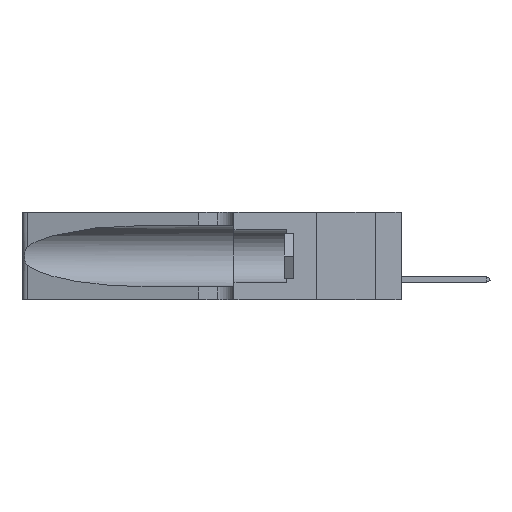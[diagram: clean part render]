
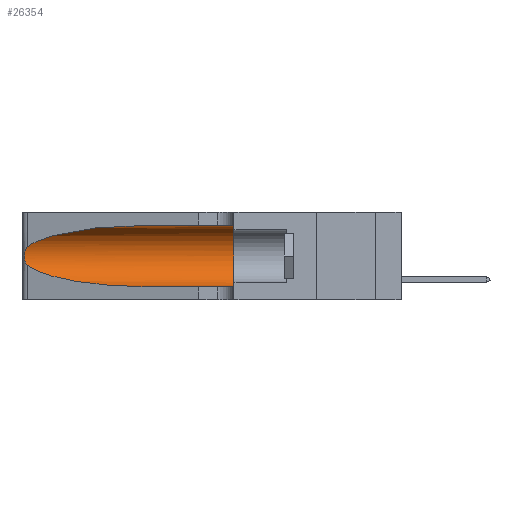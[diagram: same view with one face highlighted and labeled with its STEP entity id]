
A CAD part, left-side view. The second image highlights one B-rep face of the part: STEP entity #26354.
In plain terms, the highlighted cylindrical face has radius 3.308 mm (diameter 6.617 mm), a partial arc.
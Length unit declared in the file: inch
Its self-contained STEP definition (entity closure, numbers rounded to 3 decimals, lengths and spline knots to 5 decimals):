
#324 = CARTESIAN_POINT ( 'NONE',  ( 0.1305, 0.72297, 0.05475 ) ) ;
#990 = VERTEX_POINT ( 'NONE', #22541 ) ;
#1852 = CARTESIAN_POINT ( 'NONE',  ( 0.1305, 0.35, 0.05475 ) ) ;
#2638 = CARTESIAN_POINT ( 'NONE',  ( 0.25787, 1.23484, 0.2124 ) ) ;
#2884 = CARTESIAN_POINT ( 'NONE',  ( 0.25856, 1.23593, 0.16098 ) ) ;
#3855 = DIRECTION ( 'NONE',  ( 0., -1., 0. ) ) ;
#4485 = CARTESIAN_POINT ( 'NONE',  ( 0.25555, 1.22994, 0.2215 ) ) ;
#4563 = ORIENTED_EDGE ( 'NONE', *, *, #28167, .T. ) ;
#4845 = EDGE_CURVE ( 'NONE', #14554, #990, #24560, .T. ) ;
#5690 = CARTESIAN_POINT ( 'NONE',  ( 0.2373, 1.15595, 0.08982 ) ) ;
#6168 = EDGE_CURVE ( 'NONE', #21941, #28527, #27085, .T. ) ;
#7038 = DIRECTION ( 'NONE',  ( 0., -1., 0. ) ) ;
#8207 = CARTESIAN_POINT ( 'NONE',  ( 0.25854, 1.2359, 0.20912 ) ) ;
#8331 = CARTESIAN_POINT ( 'NONE',  ( 0.25789, 1.23486, 0.15765 ) ) ;
#8493 =( BOUNDED_CURVE ( )  B_SPLINE_CURVE ( 3, ( #10900, #5690, #18861, #324 ),
 .UNSPECIFIED., .F., .F. ) 
 B_SPLINE_CURVE_WITH_KNOTS ( ( 4, 4 ),
 ( 3.44316, 4.71239 ),
 .UNSPECIFIED. ) 
 CURVE ( )  GEOMETRIC_REPRESENTATION_ITEM ( )  RATIONAL_B_SPLINE_CURVE ( ( 1., 0.87, 0.87, 1. ) ) 
 REPRESENTATION_ITEM ( '' )  );
#8570 = EDGE_CURVE ( 'NONE', #990, #28527, #21746, .T. ) ;
#9002 = EDGE_CURVE ( 'NONE', #14554, #32942, #32631, .T. ) ;
#10900 = CARTESIAN_POINT ( 'NONE',  ( 0.25487, 1.22718, 0.14631 ) ) ;
#10949 = CARTESIAN_POINT ( 'NONE',  ( 0.26017, 1.23833, 0.17102 ) ) ;
#11962 = AXIS2_PLACEMENT_3D ( 'NONE', #34559, #15386, #34212 ) ;
#13527 = VECTOR ( 'NONE', #7038, 39.37008 ) ;
#14321 = CARTESIAN_POINT ( 'NONE',  ( 0.1305, 0.72297, 0.31525 ) ) ;
#14323 = DIRECTION ( 'NONE',  ( 0., -1., 0. ) ) ;
#14347 = VERTEX_POINT ( 'NONE', #26085 ) ;
#14361 = ORIENTED_EDGE ( 'NONE', *, *, #6168, .T. ) ;
#14522 = CARTESIAN_POINT ( 'NONE',  ( 0.25487, 1.22718, 0.22369 ) ) ;
#14554 = VERTEX_POINT ( 'NONE', #22287 ) ;
#14944 = ORIENTED_EDGE ( 'NONE', *, *, #4845, .F. ) ;
#15386 = DIRECTION ( 'NONE',  ( 0., 1., 0. ) ) ;
#16003 = ORIENTED_EDGE ( 'NONE', *, *, #30446, .T. ) ;
#17860 = CARTESIAN_POINT ( 'NONE',  ( 0.2373, 1.15595, 0.28018 ) ) ;
#17993 = CARTESIAN_POINT ( 'NONE',  ( 0.25487, 1.22718, 0.22369 ) ) ;
#18099 = CARTESIAN_POINT ( 'NONE',  ( 0.25487, 1.22718, 0.22369 ) ) ;
#18861 = CARTESIAN_POINT ( 'NONE',  ( 0.18966, 0.96281, 0.05475 ) ) ;
#19148 = CARTESIAN_POINT ( 'NONE',  ( 0.25555, 1.22993, 0.14849 ) ) ;
#19368 = FACE_OUTER_BOUND ( 'NONE', #26223, .T. ) ;
#21742 = CARTESIAN_POINT ( 'NONE',  ( 0.25639, 1.23186, 0.15144 ) ) ;
#21746 = CIRCLE ( 'NONE', #11962, 0.13025 ) ;
#21858 = CARTESIAN_POINT ( 'NONE',  ( 0.26075, 1.23896, 0.19203 ) ) ;
#21941 = VERTEX_POINT ( 'NONE', #23485 ) ;
#22287 = CARTESIAN_POINT ( 'NONE',  ( 0.1305, 0.72297, 0.31525 ) ) ;
#22541 = CARTESIAN_POINT ( 'NONE',  ( 0.1305, 0.35, 0.31525 ) ) ;
#22912 = CARTESIAN_POINT ( 'NONE',  ( 0.18966, 0.96281, 0.31525 ) ) ;
#23485 = CARTESIAN_POINT ( 'NONE',  ( 0.1305, 0.72297, 0.05475 ) ) ;
#23739 = ORIENTED_EDGE ( 'NONE', *, *, #9002, .T. ) ;
#24309 = AXIS2_PLACEMENT_3D ( 'NONE', #33160, #14323, #25452 ) ;
#24461 = CARTESIAN_POINT ( 'NONE',  ( 0.26018, 1.23835, 0.19895 ) ) ;
#24560 = LINE ( 'NONE', #28492, #13527 ) ;
#25320 = CARTESIAN_POINT ( 'NONE',  ( 0.1305, 1.61858, 0.05475 ) ) ;
#25452 = DIRECTION ( 'NONE',  ( 0., 0., -1. ) ) ;
#26085 = CARTESIAN_POINT ( 'NONE',  ( 0.25487, 1.22718, 0.14631 ) ) ;
#26167 = CARTESIAN_POINT ( 'NONE',  ( 0.25639, 1.23184, 0.21858 ) ) ;
#26223 = EDGE_LOOP ( 'NONE', ( #23739, #16003, #4563, #14361, #29602, #14944 ) ) ;
#26354 = ADVANCED_FACE ( 'NONE', ( #19368 ), #34116, .F. ) ;
#26934 = CARTESIAN_POINT ( 'NONE',  ( 0.25487, 1.22718, 0.14631 ) ) ;
#27085 = LINE ( 'NONE', #25320, #32603 ) ;
#28167 = EDGE_CURVE ( 'NONE', #14347, #21941, #8493, .T. ) ;
#28466 = B_SPLINE_CURVE_WITH_KNOTS ( 'NONE', 3,
 ( #17993, #4485, #26167, #2638, #8207, #24461, #21858, #32167, #10949, #2884, #8331, #21742, #19148, #26934 ),
 .UNSPECIFIED., .F., .F.,
 ( 4, 2, 2, 2, 2, 2, 4 ),
 ( 0., 0.00027, 0.00053, 0.00107, 0.0016, 0.00187, 0.00214 ),
 .UNSPECIFIED. ) ;
#28492 = CARTESIAN_POINT ( 'NONE',  ( 0.1305, 1.61858, 0.31525 ) ) ;
#28527 = VERTEX_POINT ( 'NONE', #1852 ) ;
#29602 = ORIENTED_EDGE ( 'NONE', *, *, #8570, .F. ) ;
#30446 = EDGE_CURVE ( 'NONE', #32942, #14347, #28466, .T. ) ;
#32167 = CARTESIAN_POINT ( 'NONE',  ( 0.26075, 1.23896, 0.178 ) ) ;
#32603 = VECTOR ( 'NONE', #3855, 39.37008 ) ;
#32631 =( BOUNDED_CURVE ( )  B_SPLINE_CURVE ( 3, ( #14321, #22912, #17860, #18099 ),
 .UNSPECIFIED., .F., .F. ) 
 B_SPLINE_CURVE_WITH_KNOTS ( ( 4, 4 ),
 ( 1.5708, 2.84003 ),
 .UNSPECIFIED. ) 
 CURVE ( )  GEOMETRIC_REPRESENTATION_ITEM ( )  RATIONAL_B_SPLINE_CURVE ( ( 1., 0.87, 0.87, 1. ) ) 
 REPRESENTATION_ITEM ( '' )  );
#32942 = VERTEX_POINT ( 'NONE', #14522 ) ;
#33160 = CARTESIAN_POINT ( 'NONE',  ( 0.1305, 1.61858, 0.185 ) ) ;
#34116 = CYLINDRICAL_SURFACE ( 'NONE', #24309, 0.13025 ) ;
#34212 = DIRECTION ( 'NONE',  ( 0., 0., 1. ) ) ;
#34559 = CARTESIAN_POINT ( 'NONE',  ( 0.1305, 0.35, 0.185 ) ) ;
